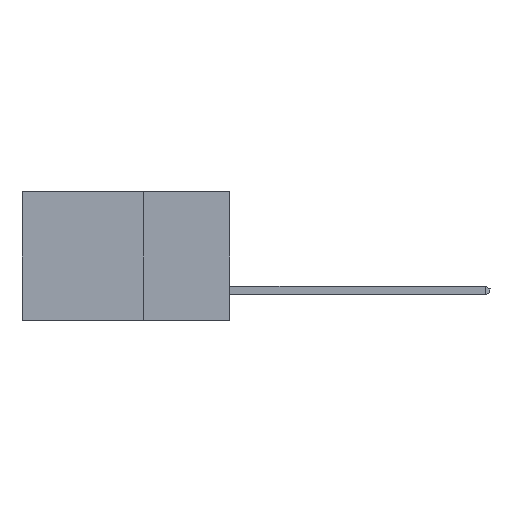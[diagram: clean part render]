
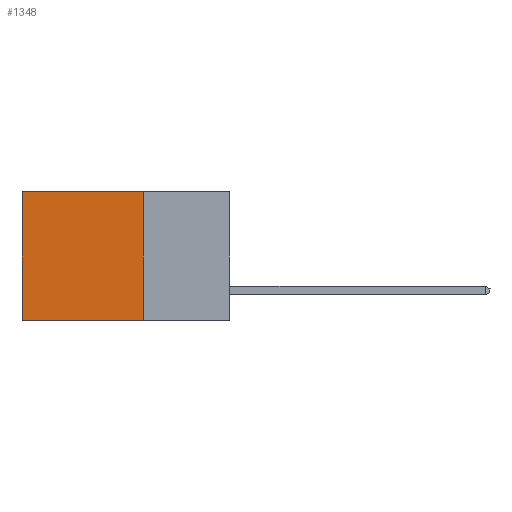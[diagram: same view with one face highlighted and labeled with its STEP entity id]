
A CAD part, left-side view. The second image highlights one B-rep face of the part: STEP entity #1348.
In plain terms, the highlighted planar face has unit normal (-1, 0, 0).
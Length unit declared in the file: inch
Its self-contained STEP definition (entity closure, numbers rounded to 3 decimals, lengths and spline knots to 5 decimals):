
#439 = CARTESIAN_POINT ( 'NONE',  ( 0.2615, 0.25, 0. ) ) ;
#446 = VERTEX_POINT ( 'NONE', #5529 ) ;
#772 = LINE ( 'NONE', #4413, #4911 ) ;
#1034 = VERTEX_POINT ( 'NONE', #7161 ) ;
#1348 = ADVANCED_FACE ( 'NONE', ( #2430 ), #3363, .F. ) ;
#2394 = VECTOR ( 'NONE', #8999, 39.37008 ) ;
#2430 = FACE_OUTER_BOUND ( 'NONE', #4284, .T. ) ;
#2666 = LINE ( 'NONE', #439, #4021 ) ;
#2836 = LINE ( 'NONE', #5112, #7083 ) ;
#2971 = DIRECTION ( 'NONE',  ( 0., 0., -1. ) ) ;
#3252 = CARTESIAN_POINT ( 'NONE',  ( 0.2615, 0.25, -0.37 ) ) ;
#3363 = PLANE ( 'NONE',  #8160 ) ;
#4002 = LINE ( 'NONE', #3252, #2394 ) ;
#4021 = VECTOR ( 'NONE', #7966, 39.37008 ) ;
#4284 = EDGE_LOOP ( 'NONE', ( #9068, #5164, #6704, #8573 ) ) ;
#4413 = CARTESIAN_POINT ( 'NONE',  ( 0.2615, 0.6, -0.37 ) ) ;
#4587 = CARTESIAN_POINT ( 'NONE',  ( 0.2615, 0.6, -0.37 ) ) ;
#4911 = VECTOR ( 'NONE', #2971, 39.37008 ) ;
#5112 = CARTESIAN_POINT ( 'NONE',  ( 0.2615, 0.25, -0.37 ) ) ;
#5164 = ORIENTED_EDGE ( 'NONE', *, *, #8612, .F. ) ;
#5424 = CARTESIAN_POINT ( 'NONE',  ( 0.2615, 0.25, -0.37 ) ) ;
#5529 = CARTESIAN_POINT ( 'NONE',  ( 0.2615, 0.6, 0. ) ) ;
#5555 = DIRECTION ( 'NONE',  ( 1., 0., 0. ) ) ;
#5602 = CARTESIAN_POINT ( 'NONE',  ( 0.2615, 0.25, -0.37 ) ) ;
#5687 = EDGE_CURVE ( 'NONE', #1034, #5974, #2836, .T. ) ;
#5974 = VERTEX_POINT ( 'NONE', #5424 ) ;
#6381 = DIRECTION ( 'NONE',  ( 0., 0., -1. ) ) ;
#6453 = EDGE_CURVE ( 'NONE', #1034, #446, #2666, .T. ) ;
#6704 = ORIENTED_EDGE ( 'NONE', *, *, #5687, .F. ) ;
#7083 = VECTOR ( 'NONE', #6381, 39.37008 ) ;
#7161 = CARTESIAN_POINT ( 'NONE',  ( 0.2615, 0.25, 0. ) ) ;
#7966 = DIRECTION ( 'NONE',  ( 0., 1., 0. ) ) ;
#8089 = VERTEX_POINT ( 'NONE', #4587 ) ;
#8160 = AXIS2_PLACEMENT_3D ( 'NONE', #5602, #5555, #8456 ) ;
#8433 = EDGE_CURVE ( 'NONE', #446, #8089, #772, .T. ) ;
#8456 = DIRECTION ( 'NONE',  ( 0., 0., -1. ) ) ;
#8573 = ORIENTED_EDGE ( 'NONE', *, *, #6453, .T. ) ;
#8612 = EDGE_CURVE ( 'NONE', #5974, #8089, #4002, .T. ) ;
#8999 = DIRECTION ( 'NONE',  ( 0., 1., 0. ) ) ;
#9068 = ORIENTED_EDGE ( 'NONE', *, *, #8433, .T. ) ;
